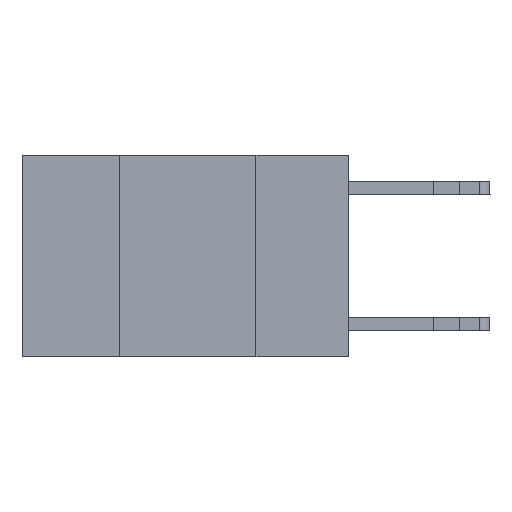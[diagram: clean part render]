
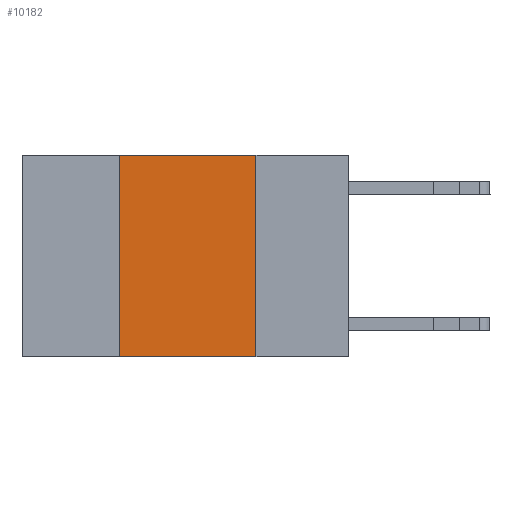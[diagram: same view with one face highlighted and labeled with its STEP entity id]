
A CAD part, left-side view. The second image highlights one B-rep face of the part: STEP entity #10182.
In plain terms, the highlighted planar face has unit normal (-1, 0, 0).
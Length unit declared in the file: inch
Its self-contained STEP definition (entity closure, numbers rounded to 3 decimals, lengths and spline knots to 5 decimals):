
#288 = DIRECTION ( 'NONE',  ( 0., 0., -1. ) ) ;
#514 = CARTESIAN_POINT ( 'NONE',  ( 0., 0.42, 0. ) ) ;
#681 = VERTEX_POINT ( 'NONE', #514 ) ;
#2263 = AXIS2_PLACEMENT_3D ( 'NONE', #4348, #17133, #288 ) ;
#2383 = CARTESIAN_POINT ( 'NONE',  ( 0., 0.42, -0.37 ) ) ;
#2889 = VECTOR ( 'NONE', #15327, 39.37008 ) ;
#3101 = EDGE_CURVE ( 'NONE', #16762, #13336, #13746, .T. ) ;
#3612 = LINE ( 'NONE', #6362, #8178 ) ;
#4348 = CARTESIAN_POINT ( 'NONE',  ( 0., 0.6, 0. ) ) ;
#4936 = CARTESIAN_POINT ( 'NONE',  ( 0., 0.42, 0. ) ) ;
#5428 = ORIENTED_EDGE ( 'NONE', *, *, #10792, .F. ) ;
#6362 = CARTESIAN_POINT ( 'NONE',  ( 0., 0.6, 0. ) ) ;
#6704 = DIRECTION ( 'NONE',  ( 0., 0., -1. ) ) ;
#6762 = VECTOR ( 'NONE', #6704, 39.37008 ) ;
#6986 = VECTOR ( 'NONE', #16081, 39.37008 ) ;
#7257 = CARTESIAN_POINT ( 'NONE',  ( 0., 0.17, -0.37 ) ) ;
#7862 = EDGE_CURVE ( 'NONE', #16182, #13336, #17890, .T. ) ;
#8178 = VECTOR ( 'NONE', #11831, 39.37008 ) ;
#8284 = CARTESIAN_POINT ( 'NONE',  ( 0., 0.17, 0. ) ) ;
#10182 = ADVANCED_FACE ( 'NONE', ( #17042 ), #10209, .F. ) ;
#10209 = PLANE ( 'NONE',  #2263 ) ;
#10792 = EDGE_CURVE ( 'NONE', #16182, #681, #13258, .T. ) ;
#10968 = CARTESIAN_POINT ( 'NONE',  ( 0., 0.6, -0.37 ) ) ;
#11617 = EDGE_CURVE ( 'NONE', #681, #16762, #3612, .T. ) ;
#11831 = DIRECTION ( 'NONE',  ( 0., -1., 0. ) ) ;
#12537 = ORIENTED_EDGE ( 'NONE', *, *, #7862, .T. ) ;
#13258 = LINE ( 'NONE', #4936, #6986 ) ;
#13336 = VERTEX_POINT ( 'NONE', #7257 ) ;
#13579 = ORIENTED_EDGE ( 'NONE', *, *, #11617, .F. ) ;
#13746 = LINE ( 'NONE', #8284, #6762 ) ;
#14046 = ORIENTED_EDGE ( 'NONE', *, *, #3101, .F. ) ;
#15327 = DIRECTION ( 'NONE',  ( 0., -1., 0. ) ) ;
#16081 = DIRECTION ( 'NONE',  ( 0., 0., 1. ) ) ;
#16182 = VERTEX_POINT ( 'NONE', #2383 ) ;
#16626 = CARTESIAN_POINT ( 'NONE',  ( 0., 0.17, 0. ) ) ;
#16762 = VERTEX_POINT ( 'NONE', #16626 ) ;
#17042 = FACE_OUTER_BOUND ( 'NONE', #17661, .T. ) ;
#17133 = DIRECTION ( 'NONE',  ( 1., 0., 0. ) ) ;
#17661 = EDGE_LOOP ( 'NONE', ( #14046, #13579, #5428, #12537 ) ) ;
#17890 = LINE ( 'NONE', #10968, #2889 ) ;
